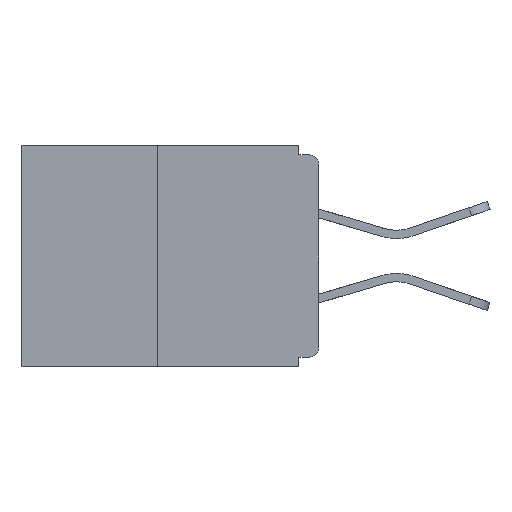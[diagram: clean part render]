
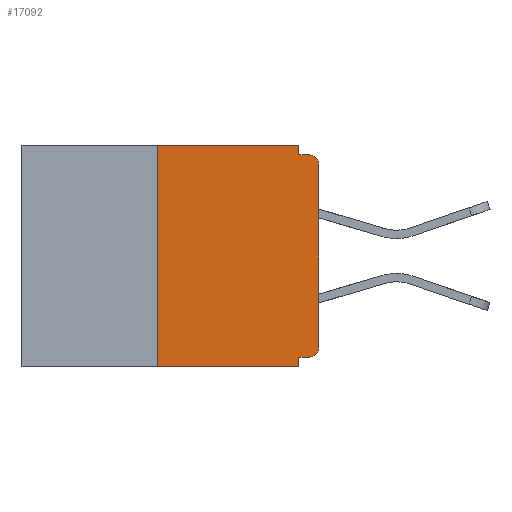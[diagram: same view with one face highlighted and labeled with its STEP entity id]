
A CAD part, left-side view. The second image highlights one B-rep face of the part: STEP entity #17092.
In plain terms, the highlighted planar face has unit normal (-1, 0, 0).
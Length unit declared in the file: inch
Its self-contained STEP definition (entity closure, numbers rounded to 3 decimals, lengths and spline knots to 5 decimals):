
#98 = DIRECTION ( 'NONE',  ( -1., 0., 0. ) ) ;
#247 = EDGE_CURVE ( 'NONE', #6758, #11997, #11209, .T. ) ;
#308 = CARTESIAN_POINT ( 'NONE',  ( 0., 0., -0.328 ) ) ;
#1112 = LINE ( 'NONE', #11483, #1660 ) ;
#1426 = EDGE_CURVE ( 'NONE', #11997, #16371, #7388, .T. ) ;
#1660 = VECTOR ( 'NONE', #14779, 39.37008 ) ;
#1684 = CARTESIAN_POINT ( 'NONE',  ( 0., 0.25, 0. ) ) ;
#1884 = EDGE_LOOP ( 'NONE', ( #6497, #19525, #6416, #16130, #14405, #19426, #2177, #12304, #9055, #5865 ) ) ;
#2014 = DIRECTION ( 'NONE',  ( 0., 0., -1. ) ) ;
#2177 = ORIENTED_EDGE ( 'NONE', *, *, #6850, .T. ) ;
#2402 = LINE ( 'NONE', #4730, #5385 ) ;
#2587 = CARTESIAN_POINT ( 'NONE',  ( 0., 0.015, -0.328 ) ) ;
#3011 = CARTESIAN_POINT ( 'NONE',  ( 0., 0.031, -0.343 ) ) ;
#3879 = DIRECTION ( 'NONE',  ( -1., 0., 0. ) ) ;
#4235 = VECTOR ( 'NONE', #13578, 39.37008 ) ;
#4293 = AXIS2_PLACEMENT_3D ( 'NONE', #6779, #10082, #22187 ) ;
#4730 = CARTESIAN_POINT ( 'NONE',  ( 0., 0.25, 0. ) ) ;
#4739 = EDGE_CURVE ( 'NONE', #22159, #6758, #2402, .T. ) ;
#4742 = CIRCLE ( 'NONE', #17537, 0.015 ) ;
#4822 = EDGE_CURVE ( 'NONE', #21573, #15665, #10987, .T. ) ;
#5079 = VECTOR ( 'NONE', #8401, 39.37008 ) ;
#5181 = CARTESIAN_POINT ( 'NONE',  ( 0., 0.031, -0.328 ) ) ;
#5385 = VECTOR ( 'NONE', #18386, 39.37008 ) ;
#5400 = CARTESIAN_POINT ( 'NONE',  ( 0., 0.015, -0.313 ) ) ;
#5544 = LINE ( 'NONE', #308, #9537 ) ;
#5576 = EDGE_CURVE ( 'NONE', #22159, #13815, #15797, .T. ) ;
#5865 = ORIENTED_EDGE ( 'NONE', *, *, #1426, .F. ) ;
#5987 = CARTESIAN_POINT ( 'NONE',  ( 0., 0.031, -0.343 ) ) ;
#6367 = EDGE_CURVE ( 'NONE', #10217, #19614, #4742, .T. ) ;
#6416 = ORIENTED_EDGE ( 'NONE', *, *, #5576, .T. ) ;
#6497 = ORIENTED_EDGE ( 'NONE', *, *, #247, .F. ) ;
#6758 = VERTEX_POINT ( 'NONE', #1684 ) ;
#6779 = CARTESIAN_POINT ( 'NONE',  ( 0., 0.46, 0. ) ) ;
#6850 = EDGE_CURVE ( 'NONE', #19614, #21573, #8186, .T. ) ;
#7388 = LINE ( 'NONE', #14567, #18964 ) ;
#8186 = LINE ( 'NONE', #19406, #17349 ) ;
#8401 = DIRECTION ( 'NONE',  ( 0., 0., -1. ) ) ;
#8440 = CARTESIAN_POINT ( 'NONE',  ( 0., 0.46, -0.343 ) ) ;
#9055 = ORIENTED_EDGE ( 'NONE', *, *, #9310, .F. ) ;
#9058 = DIRECTION ( 'NONE',  ( 0., 0., -1. ) ) ;
#9231 = CARTESIAN_POINT ( 'NONE',  ( 0., 0.031, -0.015 ) ) ;
#9310 = EDGE_CURVE ( 'NONE', #16371, #15665, #1112, .T. ) ;
#9329 = VECTOR ( 'NONE', #17355, 39.37008 ) ;
#9537 = VECTOR ( 'NONE', #12484, 39.37008 ) ;
#10082 = DIRECTION ( 'NONE',  ( 1., 0., 0. ) ) ;
#10217 = VERTEX_POINT ( 'NONE', #2587 ) ;
#10968 = FACE_OUTER_BOUND ( 'NONE', #1884, .T. ) ;
#10987 = CIRCLE ( 'NONE', #12062, 0.015 ) ;
#11209 = LINE ( 'NONE', #19031, #9329 ) ;
#11309 = DIRECTION ( 'NONE',  ( 0., 0., -1. ) ) ;
#11483 = CARTESIAN_POINT ( 'NONE',  ( 0., 0., -0.015 ) ) ;
#11982 = CARTESIAN_POINT ( 'NONE',  ( 0., 0., -0.313 ) ) ;
#11997 = VERTEX_POINT ( 'NONE', #13016 ) ;
#12062 = AXIS2_PLACEMENT_3D ( 'NONE', #15901, #3879, #9058 ) ;
#12251 = EDGE_CURVE ( 'NONE', #20397, #13815, #19850, .T. ) ;
#12304 = ORIENTED_EDGE ( 'NONE', *, *, #4822, .T. ) ;
#12484 = DIRECTION ( 'NONE',  ( 0., 1., 0. ) ) ;
#13016 = CARTESIAN_POINT ( 'NONE',  ( 0., 0.031, 0. ) ) ;
#13578 = DIRECTION ( 'NONE',  ( 0., -1., 0. ) ) ;
#13815 = VERTEX_POINT ( 'NONE', #5987 ) ;
#14115 = DIRECTION ( 'NONE',  ( 0., 0., 1. ) ) ;
#14405 = ORIENTED_EDGE ( 'NONE', *, *, #18734, .F. ) ;
#14567 = CARTESIAN_POINT ( 'NONE',  ( 0., 0.031, 0. ) ) ;
#14779 = DIRECTION ( 'NONE',  ( 0., -1., 0. ) ) ;
#15185 = PLANE ( 'NONE',  #4293 ) ;
#15220 = CARTESIAN_POINT ( 'NONE',  ( 0., 0.25, -0.343 ) ) ;
#15665 = VERTEX_POINT ( 'NONE', #21258 ) ;
#15797 = LINE ( 'NONE', #8440, #4235 ) ;
#15901 = CARTESIAN_POINT ( 'NONE',  ( 0., 0.015, -0.03 ) ) ;
#16130 = ORIENTED_EDGE ( 'NONE', *, *, #12251, .F. ) ;
#16371 = VERTEX_POINT ( 'NONE', #9231 ) ;
#16938 = CARTESIAN_POINT ( 'NONE',  ( 0., 0., -0.03 ) ) ;
#17092 = ADVANCED_FACE ( 'NONE', ( #10968 ), #15185, .F. ) ;
#17349 = VECTOR ( 'NONE', #14115, 39.37008 ) ;
#17355 = DIRECTION ( 'NONE',  ( 0., -1., 0. ) ) ;
#17537 = AXIS2_PLACEMENT_3D ( 'NONE', #5400, #98, #2014 ) ;
#18386 = DIRECTION ( 'NONE',  ( 0., 0., 1. ) ) ;
#18734 = EDGE_CURVE ( 'NONE', #10217, #20397, #5544, .T. ) ;
#18964 = VECTOR ( 'NONE', #11309, 39.37008 ) ;
#19031 = CARTESIAN_POINT ( 'NONE',  ( 0., 0.46, 0. ) ) ;
#19406 = CARTESIAN_POINT ( 'NONE',  ( 0., 0., 0. ) ) ;
#19426 = ORIENTED_EDGE ( 'NONE', *, *, #6367, .T. ) ;
#19525 = ORIENTED_EDGE ( 'NONE', *, *, #4739, .F. ) ;
#19614 = VERTEX_POINT ( 'NONE', #11982 ) ;
#19850 = LINE ( 'NONE', #3011, #5079 ) ;
#20397 = VERTEX_POINT ( 'NONE', #5181 ) ;
#21258 = CARTESIAN_POINT ( 'NONE',  ( 0., 0.015, -0.015 ) ) ;
#21573 = VERTEX_POINT ( 'NONE', #16938 ) ;
#22159 = VERTEX_POINT ( 'NONE', #15220 ) ;
#22187 = DIRECTION ( 'NONE',  ( 0., 0., -1. ) ) ;
